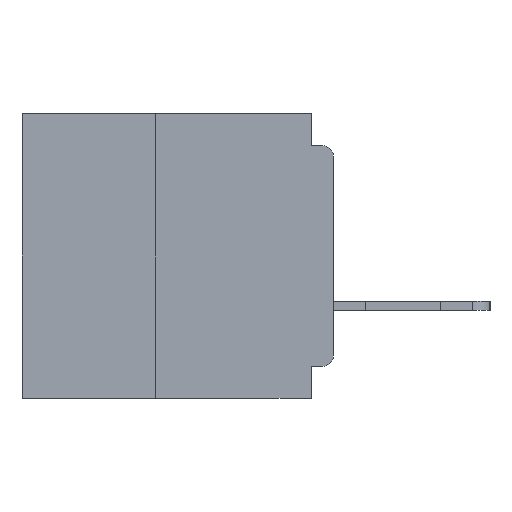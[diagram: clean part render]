
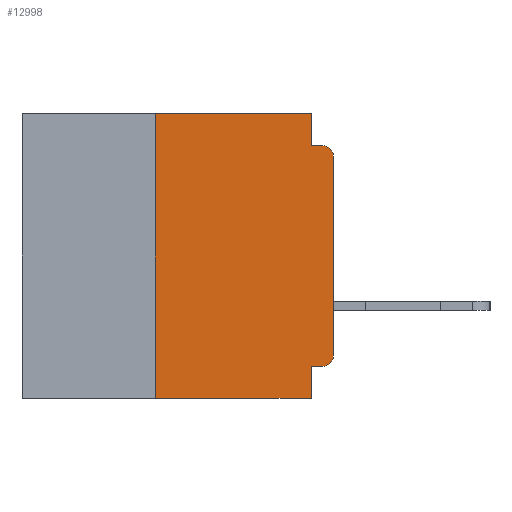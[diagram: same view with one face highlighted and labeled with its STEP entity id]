
A CAD part, left-side view. The second image highlights one B-rep face of the part: STEP entity #12998.
In plain terms, the highlighted planar face has unit normal (-1, 0, 0).
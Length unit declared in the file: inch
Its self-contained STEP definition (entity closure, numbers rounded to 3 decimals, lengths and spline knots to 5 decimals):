
#831 = LINE ( 'NONE', #35981, #17683 ) ;
#1029 = CARTESIAN_POINT ( 'NONE',  ( 0., 0.031, -0.4 ) ) ;
#1203 = CARTESIAN_POINT ( 'NONE',  ( 0., 0.015, -0.355 ) ) ;
#1249 = LINE ( 'NONE', #41948, #11532 ) ;
#3497 = CIRCLE ( 'NONE', #16657, 0.015 ) ;
#3500 = VERTEX_POINT ( 'NONE', #34397 ) ;
#3675 = DIRECTION ( 'NONE',  ( 0., 0., 1. ) ) ;
#3892 = ORIENTED_EDGE ( 'NONE', *, *, #44865, .T. ) ;
#4511 = AXIS2_PLACEMENT_3D ( 'NONE', #38982, #16085, #42738 ) ;
#5825 = EDGE_CURVE ( 'NONE', #21411, #27622, #43433, .T. ) ;
#6117 = DIRECTION ( 'NONE',  ( 0., 0., 1. ) ) ;
#6220 = FACE_OUTER_BOUND ( 'NONE', #45116, .T. ) ;
#6442 = CARTESIAN_POINT ( 'NONE',  ( 0., 0.015, -0.045 ) ) ;
#6962 = DIRECTION ( 'NONE',  ( 0., -1., 0. ) ) ;
#7435 = EDGE_CURVE ( 'NONE', #27622, #19973, #29944, .T. ) ;
#8808 = DIRECTION ( 'NONE',  ( 0., 0., -1. ) ) ;
#9321 = CARTESIAN_POINT ( 'NONE',  ( 0., 0.015, -0.06 ) ) ;
#9408 = ORIENTED_EDGE ( 'NONE', *, *, #38592, .T. ) ;
#9511 = DIRECTION ( 'NONE',  ( 0., 1., 0. ) ) ;
#9679 = CARTESIAN_POINT ( 'NONE',  ( 0., 0.031, -0.4 ) ) ;
#9709 = CIRCLE ( 'NONE', #4511, 0.015 ) ;
#10584 = DIRECTION ( 'NONE',  ( 0., 0., -1. ) ) ;
#10847 = CARTESIAN_POINT ( 'NONE',  ( 0., 0.437, 0. ) ) ;
#11532 = VECTOR ( 'NONE', #3675, 39.37008 ) ;
#11636 = CARTESIAN_POINT ( 'NONE',  ( 0., 0.031, -0.355 ) ) ;
#12191 = CARTESIAN_POINT ( 'NONE',  ( 0., 0., -0.06 ) ) ;
#12690 = CARTESIAN_POINT ( 'NONE',  ( 0., 0.25, 0. ) ) ;
#12998 = ADVANCED_FACE ( 'NONE', ( #6220 ), #39101, .F. ) ;
#13192 = DIRECTION ( 'NONE',  ( 0., 0., -1. ) ) ;
#13540 = CARTESIAN_POINT ( 'NONE',  ( 0., 0., -0.355 ) ) ;
#13984 = EDGE_CURVE ( 'NONE', #36632, #16619, #1249, .T. ) ;
#14151 = EDGE_CURVE ( 'NONE', #3500, #19973, #33676, .T. ) ;
#15229 = VECTOR ( 'NONE', #6117, 39.37008 ) ;
#16085 = DIRECTION ( 'NONE',  ( -1., 0., 0. ) ) ;
#16428 = DIRECTION ( 'NONE',  ( 0., -1., 0. ) ) ;
#16619 = VERTEX_POINT ( 'NONE', #12191 ) ;
#16657 = AXIS2_PLACEMENT_3D ( 'NONE', #9321, #36126, #13192 ) ;
#17683 = VECTOR ( 'NONE', #39767, 39.37008 ) ;
#17735 = ORIENTED_EDGE ( 'NONE', *, *, #17962, .F. ) ;
#17962 = EDGE_CURVE ( 'NONE', #42039, #21685, #831, .T. ) ;
#18412 = ORIENTED_EDGE ( 'NONE', *, *, #5825, .F. ) ;
#19729 = VECTOR ( 'NONE', #8808, 39.37008 ) ;
#19973 = VERTEX_POINT ( 'NONE', #9679 ) ;
#20067 = DIRECTION ( 'NONE',  ( 0., 0., -1. ) ) ;
#20133 = CARTESIAN_POINT ( 'NONE',  ( 0., 0.437, -0.4 ) ) ;
#21411 = VERTEX_POINT ( 'NONE', #1203 ) ;
#21458 = VERTEX_POINT ( 'NONE', #28276 ) ;
#21685 = VERTEX_POINT ( 'NONE', #6442 ) ;
#22178 = VECTOR ( 'NONE', #6962, 39.37008 ) ;
#23039 = CARTESIAN_POINT ( 'NONE',  ( 0., 0.031, 0. ) ) ;
#23678 = EDGE_CURVE ( 'NONE', #21458, #42039, #32957, .T. ) ;
#23745 = ORIENTED_EDGE ( 'NONE', *, *, #30378, .F. ) ;
#27594 = CARTESIAN_POINT ( 'NONE',  ( 0., 0.437, 0. ) ) ;
#27622 = VERTEX_POINT ( 'NONE', #11636 ) ;
#27811 = CARTESIAN_POINT ( 'NONE',  ( 0., 0., -0.34 ) ) ;
#28276 = CARTESIAN_POINT ( 'NONE',  ( 0., 0.031, 0. ) ) ;
#29944 = LINE ( 'NONE', #1029, #19729 ) ;
#30248 = AXIS2_PLACEMENT_3D ( 'NONE', #27594, #42856, #20067 ) ;
#30378 = EDGE_CURVE ( 'NONE', #35495, #21458, #42423, .T. ) ;
#32957 = LINE ( 'NONE', #23039, #33457 ) ;
#33457 = VECTOR ( 'NONE', #10584, 39.37008 ) ;
#33676 = LINE ( 'NONE', #20133, #43728 ) ;
#34397 = CARTESIAN_POINT ( 'NONE',  ( 0., 0.25, -0.4 ) ) ;
#34604 = VECTOR ( 'NONE', #9511, 39.37008 ) ;
#35495 = VERTEX_POINT ( 'NONE', #12690 ) ;
#35981 = CARTESIAN_POINT ( 'NONE',  ( 0., 0., -0.045 ) ) ;
#36126 = DIRECTION ( 'NONE',  ( -1., 0., 0. ) ) ;
#36614 = CARTESIAN_POINT ( 'NONE',  ( 0., 0.25, -0.4 ) ) ;
#36632 = VERTEX_POINT ( 'NONE', #27811 ) ;
#37357 = EDGE_CURVE ( 'NONE', #3500, #35495, #37979, .T. ) ;
#37979 = LINE ( 'NONE', #36614, #15229 ) ;
#38079 = ORIENTED_EDGE ( 'NONE', *, *, #23678, .F. ) ;
#38123 = CARTESIAN_POINT ( 'NONE',  ( 0., 0.031, -0.045 ) ) ;
#38592 = EDGE_CURVE ( 'NONE', #21411, #36632, #9709, .T. ) ;
#38982 = CARTESIAN_POINT ( 'NONE',  ( 0., 0.015, -0.34 ) ) ;
#39101 = PLANE ( 'NONE',  #30248 ) ;
#39767 = DIRECTION ( 'NONE',  ( 0., -1., 0. ) ) ;
#40990 = ORIENTED_EDGE ( 'NONE', *, *, #13984, .T. ) ;
#41948 = CARTESIAN_POINT ( 'NONE',  ( 0., 0., 0. ) ) ;
#42039 = VERTEX_POINT ( 'NONE', #38123 ) ;
#42423 = LINE ( 'NONE', #10847, #22178 ) ;
#42738 = DIRECTION ( 'NONE',  ( 0., 0., -1. ) ) ;
#42856 = DIRECTION ( 'NONE',  ( 1., 0., 0. ) ) ;
#43433 = LINE ( 'NONE', #13540, #34604 ) ;
#43728 = VECTOR ( 'NONE', #16428, 39.37008 ) ;
#44865 = EDGE_CURVE ( 'NONE', #16619, #21685, #3497, .T. ) ;
#45116 = EDGE_LOOP ( 'NONE', ( #40990, #3892, #17735, #38079, #23745, #46913, #48091, #45201, #18412, #9408 ) ) ;
#45201 = ORIENTED_EDGE ( 'NONE', *, *, #7435, .F. ) ;
#46913 = ORIENTED_EDGE ( 'NONE', *, *, #37357, .F. ) ;
#48091 = ORIENTED_EDGE ( 'NONE', *, *, #14151, .T. ) ;
